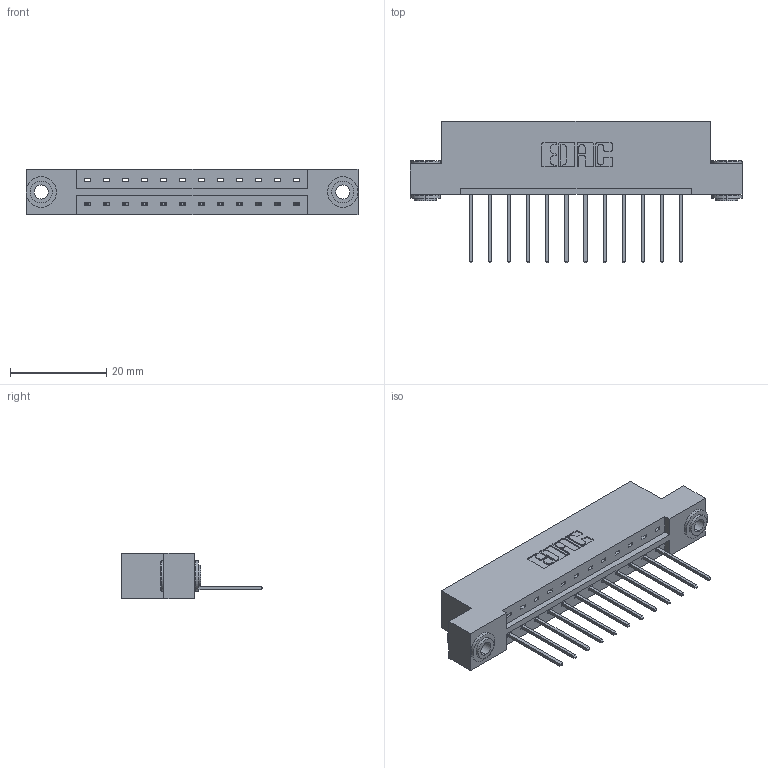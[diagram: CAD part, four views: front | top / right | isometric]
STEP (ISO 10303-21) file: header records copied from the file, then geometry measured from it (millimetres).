
FILE_DESCRIPTION (( 'STEP AP203' ), '1' );
FILE_NAME ('833-012-540-103.STEP', '2020-05-30T21:37:07', ( '' ), ( '' ), 'SwSTEP 2.0', 'SolidWorks 2020', '' );
FILE_SCHEMA (( 'CONFIG_CONTROL_DESIGN' ));
Length unit declared in the file: inch
Products named in the file (4): 833-012-540-103; 345-250-002_345-250-002-102; 345-292-001_345-293-140; 833 Part_Flush - .156 Dia - TH
Assembly tree (15 placements, depth 2):
  833-012-540-103
    833 Part_Flush - .156 Dia - TH
    345-292-001_345-293-140  x12
    345-250-002_345-250-002-102  x2
Bounding box: 69.09 x 29.47 x 9.4 mm (x, y, z)
Volume: 6729.8 mm3; surface area: 7434.1 mm2
Topology: 15 solids, 15 shells, 848 faces, 2499 edges, 1646 vertices
Faces by surface type: plane 584, cylinder 256, cone 8
Entity records: 11884 total; most frequent: CARTESIAN_POINT 2033, ORIENTED_EDGE 1974, DIRECTION 1809, EDGE_CURVE 987, LINE 835, VECTOR 835, VERTEX_POINT 654, AXIS2_PLACEMENT_3D 487
